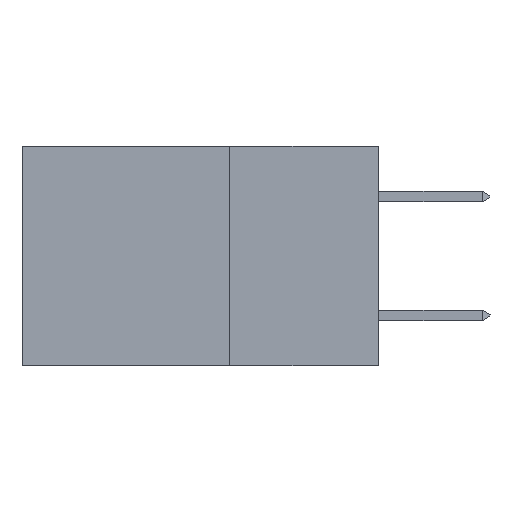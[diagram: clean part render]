
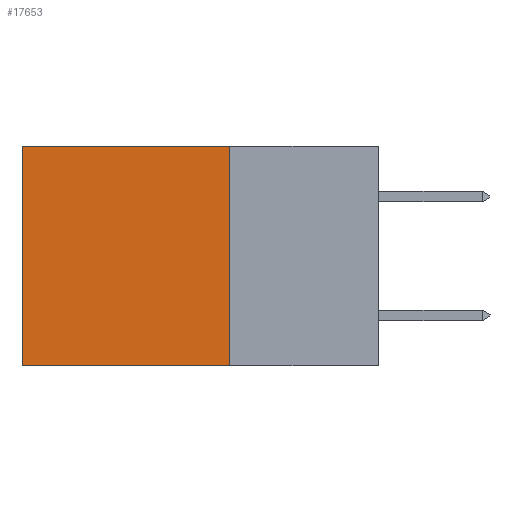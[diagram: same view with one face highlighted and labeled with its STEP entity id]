
A CAD part, left-side view. The second image highlights one B-rep face of the part: STEP entity #17653.
In plain terms, the highlighted planar face has unit normal (-1, 0, 0).
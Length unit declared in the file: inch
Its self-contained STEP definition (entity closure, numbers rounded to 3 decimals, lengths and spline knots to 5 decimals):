
#2626 = AXIS2_PLACEMENT_3D ( 'NONE', #16217, #13769, #31304 ) ;
#3004 = EDGE_CURVE ( 'NONE', #22562, #30210, #4459, .T. ) ;
#4459 = LINE ( 'NONE', #24854, #6039 ) ;
#6039 = VECTOR ( 'NONE', #17150, 39.37008 ) ;
#7066 = CARTESIAN_POINT ( 'NONE',  ( 0.298, 0.25, 0. ) ) ;
#9613 = DIRECTION ( 'NONE',  ( 0., 1., 0. ) ) ;
#9977 = VERTEX_POINT ( 'NONE', #13565 ) ;
#11058 = CARTESIAN_POINT ( 'NONE',  ( 0.298, 0.25, -0.37 ) ) ;
#13040 = VECTOR ( 'NONE', #9613, 39.37008 ) ;
#13565 = CARTESIAN_POINT ( 'NONE',  ( 0.298, 0.25, 0. ) ) ;
#13769 = DIRECTION ( 'NONE',  ( 1., 0., 0. ) ) ;
#13842 = LINE ( 'NONE', #7066, #13040 ) ;
#15504 = CARTESIAN_POINT ( 'NONE',  ( 0.298, 0.25, 0. ) ) ;
#16217 = CARTESIAN_POINT ( 'NONE',  ( 0.298, 0.25, 0. ) ) ;
#17150 = DIRECTION ( 'NONE',  ( 0., 1., 0. ) ) ;
#17653 = ADVANCED_FACE ( 'NONE', ( #19932 ), #23775, .F. ) ;
#18040 = LINE ( 'NONE', #32502, #30565 ) ;
#19932 = FACE_OUTER_BOUND ( 'NONE', #25442, .T. ) ;
#20529 = DIRECTION ( 'NONE',  ( 0., 0., -1. ) ) ;
#22510 = ORIENTED_EDGE ( 'NONE', *, *, #28337, .F. ) ;
#22562 = VERTEX_POINT ( 'NONE', #11058 ) ;
#22572 = DIRECTION ( 'NONE',  ( 0., 0., -1. ) ) ;
#23775 = PLANE ( 'NONE',  #2626 ) ;
#24146 = ORIENTED_EDGE ( 'NONE', *, *, #30124, .T. ) ;
#24854 = CARTESIAN_POINT ( 'NONE',  ( 0.298, 0.25, -0.37 ) ) ;
#24907 = EDGE_CURVE ( 'NONE', #26252, #30210, #18040, .T. ) ;
#25442 = EDGE_LOOP ( 'NONE', ( #28241, #32099, #22510, #24146 ) ) ;
#26252 = VERTEX_POINT ( 'NONE', #27235 ) ;
#27235 = CARTESIAN_POINT ( 'NONE',  ( 0.298, 0.6, 0. ) ) ;
#28241 = ORIENTED_EDGE ( 'NONE', *, *, #24907, .T. ) ;
#28337 = EDGE_CURVE ( 'NONE', #9977, #22562, #29314, .T. ) ;
#28526 = VECTOR ( 'NONE', #20529, 39.37008 ) ;
#29314 = LINE ( 'NONE', #15504, #28526 ) ;
#30124 = EDGE_CURVE ( 'NONE', #9977, #26252, #13842, .T. ) ;
#30199 = CARTESIAN_POINT ( 'NONE',  ( 0.298, 0.6, -0.37 ) ) ;
#30210 = VERTEX_POINT ( 'NONE', #30199 ) ;
#30565 = VECTOR ( 'NONE', #22572, 39.37008 ) ;
#31304 = DIRECTION ( 'NONE',  ( 0., 0., -1. ) ) ;
#32099 = ORIENTED_EDGE ( 'NONE', *, *, #3004, .F. ) ;
#32502 = CARTESIAN_POINT ( 'NONE',  ( 0.298, 0.6, 0. ) ) ;
